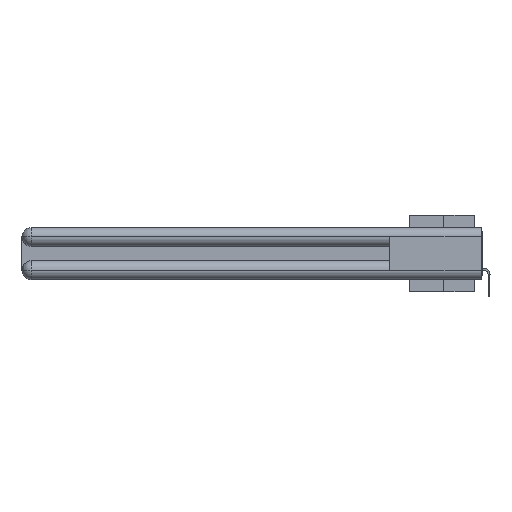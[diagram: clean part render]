
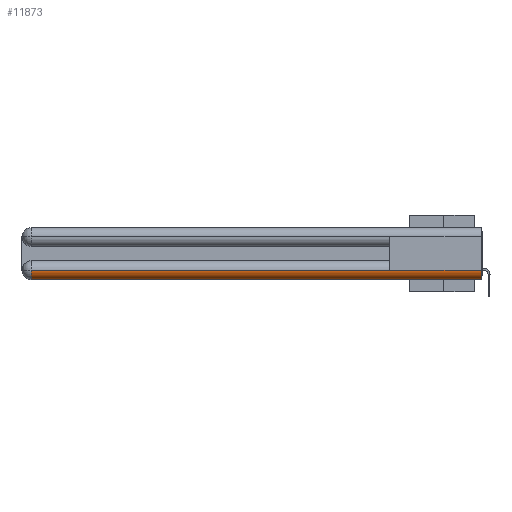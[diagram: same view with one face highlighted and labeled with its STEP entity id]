
A CAD part, left-side view. The second image highlights one B-rep face of the part: STEP entity #11873.
In plain terms, the highlighted cylindrical face has radius 1.562 mm (diameter 3.124 mm), a partial arc.
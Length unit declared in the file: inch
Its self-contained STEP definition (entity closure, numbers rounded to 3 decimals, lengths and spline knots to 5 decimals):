
#349 = CARTESIAN_POINT ( 'NONE',  ( 0.0615, 2.94, -0.34 ) ) ;
#362 = DIRECTION ( 'NONE',  ( 0., 0., -1. ) ) ;
#813 = DIRECTION ( 'NONE',  ( 0., 1., 0. ) ) ;
#1947 = CARTESIAN_POINT ( 'NONE',  ( 0.0615, 2.94, -0.2785 ) ) ;
#2379 = EDGE_CURVE ( 'NONE', #12744, #24830, #12730, .T. ) ;
#4309 = VERTEX_POINT ( 'NONE', #9929 ) ;
#4980 = EDGE_CURVE ( 'NONE', #4309, #31525, #9533, .T. ) ;
#8052 = DIRECTION ( 'NONE',  ( 0., 0., 1. ) ) ;
#8984 = FACE_OUTER_BOUND ( 'NONE', #30742, .T. ) ;
#9374 = CARTESIAN_POINT ( 'NONE',  ( 0.0615, 0., -0.2785 ) ) ;
#9533 = LINE ( 'NONE', #21498, #19540 ) ;
#9929 = CARTESIAN_POINT ( 'NONE',  ( 0., 0.6, -0.2785 ) ) ;
#11873 = ADVANCED_FACE ( 'NONE', ( #8984 ), #36063, .T. ) ;
#12730 = CIRCLE ( 'NONE', #31515, 0.0615 ) ;
#12744 = VERTEX_POINT ( 'NONE', #35962 ) ;
#12972 = LINE ( 'NONE', #24935, #24283 ) ;
#15582 = VERTEX_POINT ( 'NONE', #33095 ) ;
#16059 = ORIENTED_EDGE ( 'NONE', *, *, #37060, .F. ) ;
#16631 = LINE ( 'NONE', #25262, #22983 ) ;
#16705 = DIRECTION ( 'NONE',  ( 0., -1., 0. ) ) ;
#17284 = CARTESIAN_POINT ( 'NONE',  ( 0., 0., -0.2785 ) ) ;
#19437 = EDGE_CURVE ( 'NONE', #15582, #24830, #16631, .T. ) ;
#19506 = AXIS2_PLACEMENT_3D ( 'NONE', #9374, #21330, #362 ) ;
#19540 = VECTOR ( 'NONE', #33453, 39.37008 ) ;
#21300 = ORIENTED_EDGE ( 'NONE', *, *, #19437, .F. ) ;
#21330 = DIRECTION ( 'NONE',  ( 0., -1., 0. ) ) ;
#21498 = CARTESIAN_POINT ( 'NONE',  ( 0., 0., -0.2785 ) ) ;
#22596 = ORIENTED_EDGE ( 'NONE', *, *, #23770, .T. ) ;
#22983 = VECTOR ( 'NONE', #29174, 39.37008 ) ;
#23487 = CIRCLE ( 'NONE', #26609, 0.0615 ) ;
#23770 = EDGE_CURVE ( 'NONE', #4309, #12744, #12972, .T. ) ;
#24283 = VECTOR ( 'NONE', #813, 39.37008 ) ;
#24830 = VERTEX_POINT ( 'NONE', #349 ) ;
#24935 = CARTESIAN_POINT ( 'NONE',  ( 0., 0., -0.2785 ) ) ;
#25262 = CARTESIAN_POINT ( 'NONE',  ( 0.0615, 0., -0.34 ) ) ;
#26609 = AXIS2_PLACEMENT_3D ( 'NONE', #34188, #16705, #31409 ) ;
#29174 = DIRECTION ( 'NONE',  ( 0., 1., 0. ) ) ;
#30742 = EDGE_LOOP ( 'NONE', ( #22596, #38258, #21300, #16059, #33473 ) ) ;
#31409 = DIRECTION ( 'NONE',  ( 1., 0., 0. ) ) ;
#31515 = AXIS2_PLACEMENT_3D ( 'NONE', #1947, #38243, #8052 ) ;
#31525 = VERTEX_POINT ( 'NONE', #17284 ) ;
#33095 = CARTESIAN_POINT ( 'NONE',  ( 0.0615, 0., -0.34 ) ) ;
#33453 = DIRECTION ( 'NONE',  ( 0., -1., 0. ) ) ;
#33473 = ORIENTED_EDGE ( 'NONE', *, *, #4980, .F. ) ;
#34188 = CARTESIAN_POINT ( 'NONE',  ( 0.0615, 0., -0.2785 ) ) ;
#35962 = CARTESIAN_POINT ( 'NONE',  ( 0., 2.94, -0.2785 ) ) ;
#36063 = CYLINDRICAL_SURFACE ( 'NONE', #19506, 0.0615 ) ;
#37060 = EDGE_CURVE ( 'NONE', #31525, #15582, #23487, .T. ) ;
#38243 = DIRECTION ( 'NONE',  ( 0., -1., 0. ) ) ;
#38258 = ORIENTED_EDGE ( 'NONE', *, *, #2379, .T. ) ;
